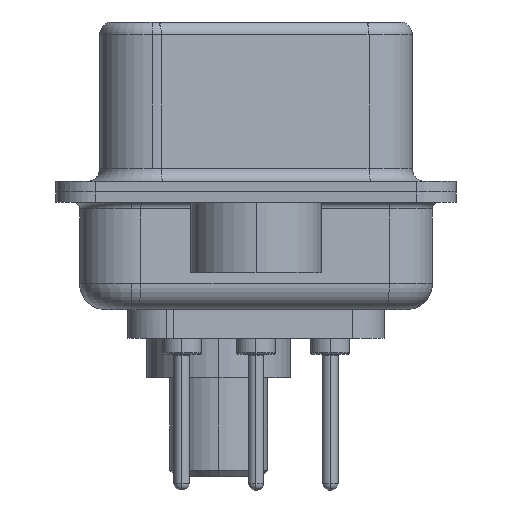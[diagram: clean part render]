
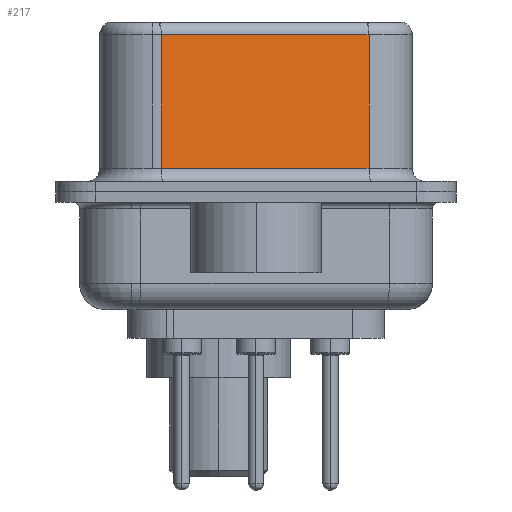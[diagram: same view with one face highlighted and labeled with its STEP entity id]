
A CAD part, left-side view. The second image highlights one B-rep face of the part: STEP entity #217.
In plain terms, the highlighted planar face has unit normal (-0.985, -0.174, 0).
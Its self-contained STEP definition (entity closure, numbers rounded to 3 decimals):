
#217 = ADVANCED_FACE ( 'NONE', ( #28805 ), #7153, .F. ) ;
#320 = CARTESIAN_POINT ( 'NONE',  ( 5.132, -4.322, 6.52 ) ) ;
#2094 = DIRECTION ( 'NONE',  ( 0., 0., -1. ) ) ;
#2785 = DIRECTION ( 'NONE',  ( -0.174, 0.985, 0. ) ) ;
#3221 = LINE ( 'NONE', #25715, #11742 ) ;
#3577 = CARTESIAN_POINT ( 'NONE',  ( 3.73, 3.628, 0.9 ) ) ;
#4581 = ORIENTED_EDGE ( 'NONE', *, *, #11031, .T. ) ;
#6458 = VERTEX_POINT ( 'NONE', #22949 ) ;
#7153 = PLANE ( 'NONE',  #21424 ) ;
#7190 = DIRECTION ( 'NONE',  ( 0.174, -0.985, 0. ) ) ;
#9065 = EDGE_CURVE ( 'NONE', #22779, #19724, #19799, .T. ) ;
#10246 = VECTOR ( 'NONE', #7190, 1000. ) ;
#11031 = EDGE_CURVE ( 'NONE', #26917, #22779, #3221, .T. ) ;
#11742 = VECTOR ( 'NONE', #19015, 1000. ) ;
#13260 = EDGE_CURVE ( 'NONE', #19724, #6458, #22726, .T. ) ;
#13261 = CARTESIAN_POINT ( 'NONE',  ( 5.132, -4.322, 6.02 ) ) ;
#16175 = EDGE_LOOP ( 'NONE', ( #29273, #4581, #19939, #27425 ) ) ;
#18481 = DIRECTION ( 'NONE',  ( 0.985, 0.174, 0. ) ) ;
#18788 = LINE ( 'NONE', #24722, #29128 ) ;
#18826 = EDGE_CURVE ( 'NONE', #26917, #6458, #18788, .T. ) ;
#19015 = DIRECTION ( 'NONE',  ( -0.174, 0.985, 0. ) ) ;
#19426 = DIRECTION ( 'NONE',  ( 0., 0., -1. ) ) ;
#19724 = VERTEX_POINT ( 'NONE', #3577 ) ;
#19799 = LINE ( 'NONE', #25899, #22294 ) ;
#19939 = ORIENTED_EDGE ( 'NONE', *, *, #9065, .T. ) ;
#21021 = CARTESIAN_POINT ( 'NONE',  ( 5.132, -4.322, 0.9 ) ) ;
#21424 = AXIS2_PLACEMENT_3D ( 'NONE', #320, #18481, #2785 ) ;
#22294 = VECTOR ( 'NONE', #19426, 1000. ) ;
#22321 = CARTESIAN_POINT ( 'NONE',  ( 3.73, 3.628, 6.02 ) ) ;
#22726 = LINE ( 'NONE', #21021, #10246 ) ;
#22779 = VERTEX_POINT ( 'NONE', #22321 ) ;
#22949 = CARTESIAN_POINT ( 'NONE',  ( 5.132, -4.322, 0.9 ) ) ;
#24722 = CARTESIAN_POINT ( 'NONE',  ( 5.132, -4.322, 6.52 ) ) ;
#25715 = CARTESIAN_POINT ( 'NONE',  ( 5.132, -4.322, 6.02 ) ) ;
#25899 = CARTESIAN_POINT ( 'NONE',  ( 3.73, 3.628, 6.52 ) ) ;
#26917 = VERTEX_POINT ( 'NONE', #13261 ) ;
#27425 = ORIENTED_EDGE ( 'NONE', *, *, #13260, .T. ) ;
#28805 = FACE_OUTER_BOUND ( 'NONE', #16175, .T. ) ;
#29128 = VECTOR ( 'NONE', #2094, 1000. ) ;
#29273 = ORIENTED_EDGE ( 'NONE', *, *, #18826, .F. ) ;
